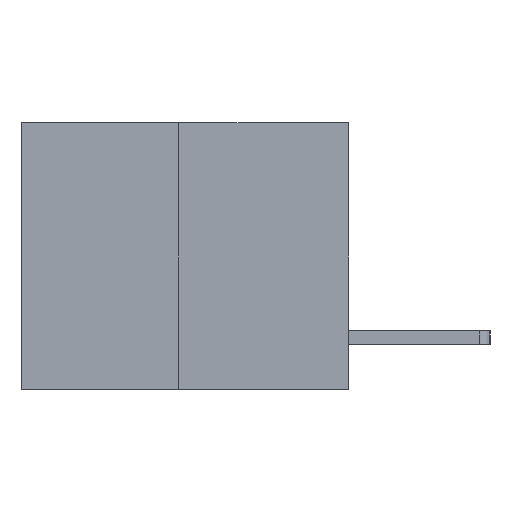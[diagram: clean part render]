
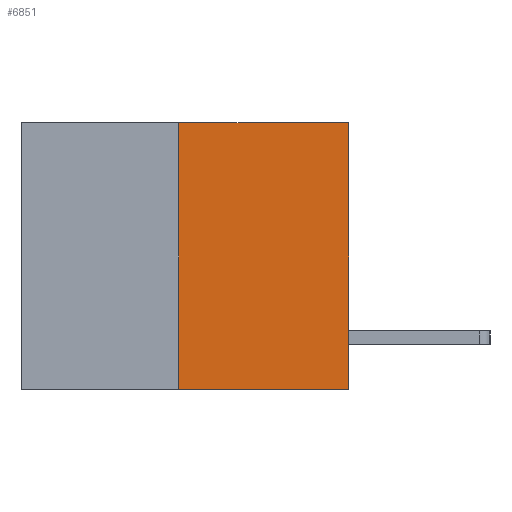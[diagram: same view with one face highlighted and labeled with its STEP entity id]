
A CAD part, left-side view. The second image highlights one B-rep face of the part: STEP entity #6851.
In plain terms, the highlighted planar face has unit normal (-1, 0, 0).
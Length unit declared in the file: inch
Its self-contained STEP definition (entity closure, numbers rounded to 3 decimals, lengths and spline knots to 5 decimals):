
#177 = ORIENTED_EDGE ( 'NONE', *, *, #7633, .T. ) ;
#236 = FACE_OUTER_BOUND ( 'NONE', #3176, .T. ) ;
#256 = LINE ( 'NONE', #5647, #7814 ) ;
#757 = LINE ( 'NONE', #782, #4566 ) ;
#782 = CARTESIAN_POINT ( 'NONE',  ( 0., 0.312, -0.49 ) ) ;
#944 = DIRECTION ( 'NONE',  ( 0., 0., -1. ) ) ;
#1247 = DIRECTION ( 'NONE',  ( 0., -1., 0. ) ) ;
#1933 = ORIENTED_EDGE ( 'NONE', *, *, #4684, .F. ) ;
#2148 = VERTEX_POINT ( 'NONE', #4619 ) ;
#2292 = AXIS2_PLACEMENT_3D ( 'NONE', #6364, #5515, #944 ) ;
#2300 = CARTESIAN_POINT ( 'NONE',  ( 0., 0.6, 0. ) ) ;
#3176 = EDGE_LOOP ( 'NONE', ( #9908, #177, #7225, #1933 ) ) ;
#3215 = DIRECTION ( 'NONE',  ( 0., -1., 0. ) ) ;
#3439 = VERTEX_POINT ( 'NONE', #5093 ) ;
#3544 = VECTOR ( 'NONE', #1247, 39.37008 ) ;
#4085 = CARTESIAN_POINT ( 'NONE',  ( 0., 0., -0.49 ) ) ;
#4123 = EDGE_CURVE ( 'NONE', #2148, #11617, #757, .T. ) ;
#4566 = VECTOR ( 'NONE', #7238, 39.37008 ) ;
#4619 = CARTESIAN_POINT ( 'NONE',  ( 0., 0.312, -0.49 ) ) ;
#4684 = EDGE_CURVE ( 'NONE', #11617, #3439, #8133, .T. ) ;
#4917 = CARTESIAN_POINT ( 'NONE',  ( 0., 0.6, -0.49 ) ) ;
#5093 = CARTESIAN_POINT ( 'NONE',  ( 0., 0., 0. ) ) ;
#5515 = DIRECTION ( 'NONE',  ( 1., 0., 0. ) ) ;
#5647 = CARTESIAN_POINT ( 'NONE',  ( 0., 0., 0. ) ) ;
#6364 = CARTESIAN_POINT ( 'NONE',  ( 0., 0.6, 0. ) ) ;
#6851 = ADVANCED_FACE ( 'NONE', ( #236 ), #11098, .F. ) ;
#6928 = VECTOR ( 'NONE', #3215, 39.37008 ) ;
#7225 = ORIENTED_EDGE ( 'NONE', *, *, #10788, .T. ) ;
#7238 = DIRECTION ( 'NONE',  ( 0., 0., 1. ) ) ;
#7633 = EDGE_CURVE ( 'NONE', #2148, #8563, #10259, .T. ) ;
#7814 = VECTOR ( 'NONE', #11406, 39.37008 ) ;
#8133 = LINE ( 'NONE', #2300, #3544 ) ;
#8563 = VERTEX_POINT ( 'NONE', #4085 ) ;
#8986 = CARTESIAN_POINT ( 'NONE',  ( 0., 0.312, 0. ) ) ;
#9908 = ORIENTED_EDGE ( 'NONE', *, *, #4123, .F. ) ;
#10259 = LINE ( 'NONE', #4917, #6928 ) ;
#10788 = EDGE_CURVE ( 'NONE', #8563, #3439, #256, .T. ) ;
#11098 = PLANE ( 'NONE',  #2292 ) ;
#11406 = DIRECTION ( 'NONE',  ( 0., 0., 1. ) ) ;
#11617 = VERTEX_POINT ( 'NONE', #8986 ) ;
